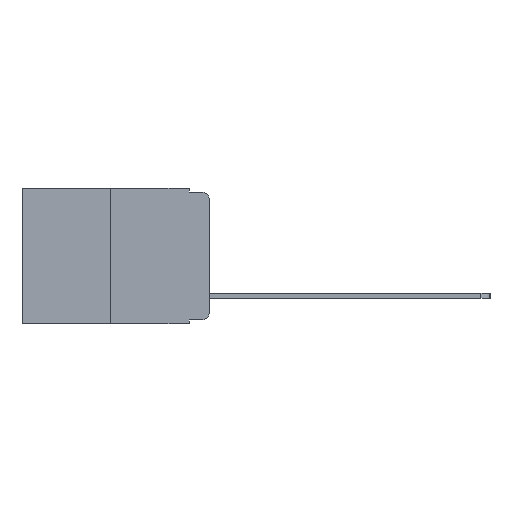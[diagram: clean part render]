
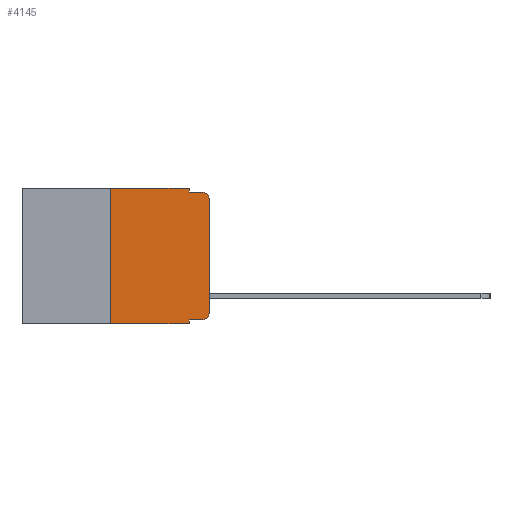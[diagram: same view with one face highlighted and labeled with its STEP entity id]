
A CAD part, left-side view. The second image highlights one B-rep face of the part: STEP entity #4145.
In plain terms, the highlighted planar face has unit normal (-1, 0, 0).
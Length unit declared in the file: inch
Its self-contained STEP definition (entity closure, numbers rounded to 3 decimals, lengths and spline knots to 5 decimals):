
#171 = CARTESIAN_POINT ( 'NONE',  ( 0., 0.02, -0.03 ) ) ;
#471 = EDGE_CURVE ( 'NONE', #1621, #1301, #7635, .T. ) ;
#492 = ORIENTED_EDGE ( 'NONE', *, *, #14977, .T. ) ;
#602 = ORIENTED_EDGE ( 'NONE', *, *, #13924, .T. ) ;
#986 = ORIENTED_EDGE ( 'NONE', *, *, #11808, .F. ) ;
#1264 = ORIENTED_EDGE ( 'NONE', *, *, #9686, .F. ) ;
#1301 = VERTEX_POINT ( 'NONE', #8155 ) ;
#1303 = ORIENTED_EDGE ( 'NONE', *, *, #2948, .F. ) ;
#1392 = CARTESIAN_POINT ( 'NONE',  ( 0., 0.473, -0.343 ) ) ;
#1395 = LINE ( 'NONE', #20965, #18247 ) ;
#1419 = VERTEX_POINT ( 'NONE', #10776 ) ;
#1621 = VERTEX_POINT ( 'NONE', #10458 ) ;
#1667 = ORIENTED_EDGE ( 'NONE', *, *, #7399, .F. ) ;
#1954 = VERTEX_POINT ( 'NONE', #9960 ) ;
#1976 = DIRECTION ( 'NONE',  ( 0., 0., -1. ) ) ;
#2148 = VERTEX_POINT ( 'NONE', #14307 ) ;
#2374 = LINE ( 'NONE', #4921, #6336 ) ;
#2394 = LINE ( 'NONE', #18653, #17508 ) ;
#2510 = VERTEX_POINT ( 'NONE', #11953 ) ;
#2529 = ORIENTED_EDGE ( 'NONE', *, *, #6083, .T. ) ;
#2634 = DIRECTION ( 'NONE',  ( 0., 0., 1. ) ) ;
#2948 = EDGE_CURVE ( 'NONE', #2148, #1954, #1395, .T. ) ;
#3137 = ORIENTED_EDGE ( 'NONE', *, *, #5067, .F. ) ;
#3474 = PLANE ( 'NONE',  #9170 ) ;
#3667 = VERTEX_POINT ( 'NONE', #6350 ) ;
#3903 = CARTESIAN_POINT ( 'NONE',  ( 0., 0.02, -0.01 ) ) ;
#3932 = EDGE_CURVE ( 'NONE', #1419, #1621, #18213, .T. ) ;
#4145 = ADVANCED_FACE ( 'NONE', ( #9633 ), #3474, .F. ) ;
#4685 = ORIENTED_EDGE ( 'NONE', *, *, #3932, .T. ) ;
#4921 = CARTESIAN_POINT ( 'NONE',  ( 0., 0.051, 0. ) ) ;
#5067 = EDGE_CURVE ( 'NONE', #1419, #2510, #2374, .T. ) ;
#5361 = VECTOR ( 'NONE', #13076, 39.37008 ) ;
#5773 = DIRECTION ( 'NONE',  ( 0., -1., 0. ) ) ;
#6083 = EDGE_CURVE ( 'NONE', #9680, #2510, #9932, .T. ) ;
#6336 = VECTOR ( 'NONE', #20941, 39.37008 ) ;
#6350 = CARTESIAN_POINT ( 'NONE',  ( 0., 0.051, -0.01 ) ) ;
#6608 = DIRECTION ( 'NONE',  ( 0., 0., -1. ) ) ;
#6651 = VERTEX_POINT ( 'NONE', #3903 ) ;
#6700 = ORIENTED_EDGE ( 'NONE', *, *, #471, .T. ) ;
#7399 = EDGE_CURVE ( 'NONE', #9680, #2148, #17271, .T. ) ;
#7635 = CIRCLE ( 'NONE', #19568, 0.02 ) ;
#8155 = CARTESIAN_POINT ( 'NONE',  ( 0., 0., -0.313 ) ) ;
#8699 = CARTESIAN_POINT ( 'NONE',  ( 0., 0.473, 0. ) ) ;
#8753 = AXIS2_PLACEMENT_3D ( 'NONE', #171, #12013, #1976 ) ;
#9170 = AXIS2_PLACEMENT_3D ( 'NONE', #8699, #19637, #10330 ) ;
#9380 = VECTOR ( 'NONE', #16067, 39.37008 ) ;
#9633 = FACE_OUTER_BOUND ( 'NONE', #11712, .T. ) ;
#9680 = VERTEX_POINT ( 'NONE', #11567 ) ;
#9686 = EDGE_CURVE ( 'NONE', #1954, #3667, #12758, .T. ) ;
#9932 = LINE ( 'NONE', #1392, #5361 ) ;
#9960 = CARTESIAN_POINT ( 'NONE',  ( 0., 0.051, 0. ) ) ;
#10330 = DIRECTION ( 'NONE',  ( 0., 0., -1. ) ) ;
#10458 = CARTESIAN_POINT ( 'NONE',  ( 0., 0.02, -0.333 ) ) ;
#10521 = VERTEX_POINT ( 'NONE', #17125 ) ;
#10776 = CARTESIAN_POINT ( 'NONE',  ( 0., 0.051, -0.333 ) ) ;
#11567 = CARTESIAN_POINT ( 'NONE',  ( 0., 0.25, -0.343 ) ) ;
#11712 = EDGE_LOOP ( 'NONE', ( #492, #602, #986, #1264, #1303, #1667, #2529, #3137, #4685, #6700 ) ) ;
#11808 = EDGE_CURVE ( 'NONE', #3667, #6651, #20896, .T. ) ;
#11953 = CARTESIAN_POINT ( 'NONE',  ( 0., 0.051, -0.343 ) ) ;
#12013 = DIRECTION ( 'NONE',  ( -1., 0., 0. ) ) ;
#12407 = DIRECTION ( 'NONE',  ( 0., 0., 1. ) ) ;
#12620 = CARTESIAN_POINT ( 'NONE',  ( 0., 0.25, 0. ) ) ;
#12758 = LINE ( 'NONE', #14737, #20017 ) ;
#13076 = DIRECTION ( 'NONE',  ( 0., -1., 0. ) ) ;
#13924 = EDGE_CURVE ( 'NONE', #10521, #6651, #14559, .T. ) ;
#13981 = CARTESIAN_POINT ( 'NONE',  ( 0., 0.051, -0.01 ) ) ;
#14099 = DIRECTION ( 'NONE',  ( 0., -1., 0. ) ) ;
#14307 = CARTESIAN_POINT ( 'NONE',  ( 0., 0.25, 0. ) ) ;
#14559 = CIRCLE ( 'NONE', #8753, 0.02 ) ;
#14564 = VECTOR ( 'NONE', #2634, 39.37008 ) ;
#14737 = CARTESIAN_POINT ( 'NONE',  ( 0., 0.051, 0. ) ) ;
#14763 = DIRECTION ( 'NONE',  ( -1., 0., 0. ) ) ;
#14977 = EDGE_CURVE ( 'NONE', #1301, #10521, #2394, .T. ) ;
#16067 = DIRECTION ( 'NONE',  ( 0., -1., 0. ) ) ;
#16350 = DIRECTION ( 'NONE',  ( 0., 0., -1. ) ) ;
#16686 = CARTESIAN_POINT ( 'NONE',  ( 0., 0.02, -0.313 ) ) ;
#17125 = CARTESIAN_POINT ( 'NONE',  ( 0., 0., -0.03 ) ) ;
#17271 = LINE ( 'NONE', #12620, #14564 ) ;
#17508 = VECTOR ( 'NONE', #12407, 39.37008 ) ;
#17632 = CARTESIAN_POINT ( 'NONE',  ( 0., 0.051, -0.333 ) ) ;
#18213 = LINE ( 'NONE', #17632, #9380 ) ;
#18247 = VECTOR ( 'NONE', #14099, 39.37008 ) ;
#18653 = CARTESIAN_POINT ( 'NONE',  ( 0., 0., 0. ) ) ;
#19568 = AXIS2_PLACEMENT_3D ( 'NONE', #16686, #14763, #16350 ) ;
#19637 = DIRECTION ( 'NONE',  ( 1., 0., 0. ) ) ;
#20017 = VECTOR ( 'NONE', #6608, 39.37008 ) ;
#20413 = VECTOR ( 'NONE', #5773, 39.37008 ) ;
#20896 = LINE ( 'NONE', #13981, #20413 ) ;
#20941 = DIRECTION ( 'NONE',  ( 0., 0., -1. ) ) ;
#20965 = CARTESIAN_POINT ( 'NONE',  ( 0., 0.473, 0. ) ) ;
